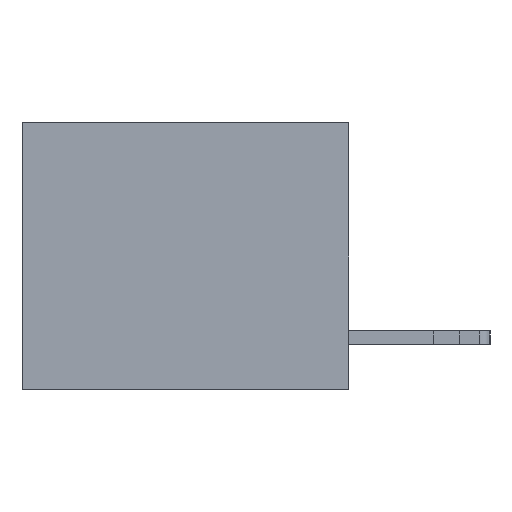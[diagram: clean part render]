
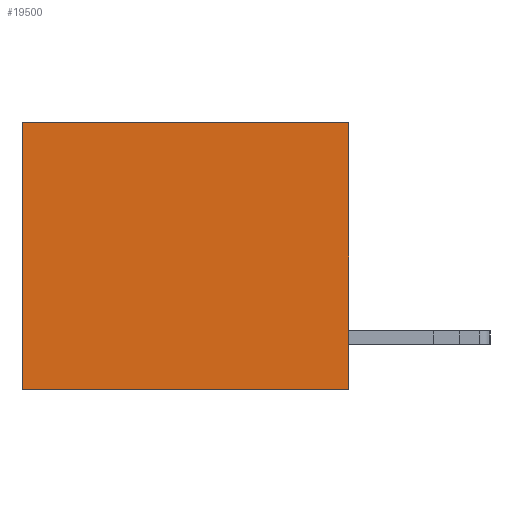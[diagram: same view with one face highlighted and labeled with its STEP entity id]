
A CAD part, left-side view. The second image highlights one B-rep face of the part: STEP entity #19500.
In plain terms, the highlighted planar face has unit normal (-1, 0, 0).
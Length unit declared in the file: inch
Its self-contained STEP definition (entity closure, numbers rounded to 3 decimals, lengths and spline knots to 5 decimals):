
#378 = DIRECTION ( 'NONE',  ( 0., 1., 0. ) ) ;
#2826 = DIRECTION ( 'NONE',  ( 1., 0., 0. ) ) ;
#3001 = CARTESIAN_POINT ( 'NONE',  ( 0.3165, 0.6, -0.49 ) ) ;
#3659 = VECTOR ( 'NONE', #4577, 39.37008 ) ;
#4577 = DIRECTION ( 'NONE',  ( 0., 0., -1. ) ) ;
#4807 = VECTOR ( 'NONE', #18859, 39.37008 ) ;
#5295 = CARTESIAN_POINT ( 'NONE',  ( 0.3165, 0.6, 0. ) ) ;
#5510 = CARTESIAN_POINT ( 'NONE',  ( 0.3165, 0., -0.49 ) ) ;
#6610 = LINE ( 'NONE', #30519, #25116 ) ;
#6663 = AXIS2_PLACEMENT_3D ( 'NONE', #5510, #2826, #17188 ) ;
#9792 = VERTEX_POINT ( 'NONE', #13735 ) ;
#12163 = LINE ( 'NONE', #23193, #4807 ) ;
#12301 = EDGE_CURVE ( 'NONE', #9792, #26466, #13832, .T. ) ;
#12869 = LINE ( 'NONE', #22359, #3659 ) ;
#13042 = ORIENTED_EDGE ( 'NONE', *, *, #18091, .T. ) ;
#13735 = CARTESIAN_POINT ( 'NONE',  ( 0.3165, 0., -0.49 ) ) ;
#13832 = LINE ( 'NONE', #24160, #20146 ) ;
#14188 = CARTESIAN_POINT ( 'NONE',  ( 0.3165, 0., 0. ) ) ;
#14693 = PLANE ( 'NONE',  #6663 ) ;
#14941 = VERTEX_POINT ( 'NONE', #14188 ) ;
#16459 = DIRECTION ( 'NONE',  ( 0., 0., -1. ) ) ;
#17188 = DIRECTION ( 'NONE',  ( 0., 0., -1. ) ) ;
#18091 = EDGE_CURVE ( 'NONE', #29698, #26466, #12869, .T. ) ;
#18859 = DIRECTION ( 'NONE',  ( 0., 1., 0. ) ) ;
#19500 = ADVANCED_FACE ( 'NONE', ( #27926 ), #14693, .F. ) ;
#19851 = EDGE_CURVE ( 'NONE', #14941, #29698, #12163, .T. ) ;
#19915 = EDGE_CURVE ( 'NONE', #14941, #9792, #6610, .T. ) ;
#20146 = VECTOR ( 'NONE', #378, 39.37008 ) ;
#22359 = CARTESIAN_POINT ( 'NONE',  ( 0.3165, 0.6, -0.49 ) ) ;
#23193 = CARTESIAN_POINT ( 'NONE',  ( 0.3165, 0., 0. ) ) ;
#24160 = CARTESIAN_POINT ( 'NONE',  ( 0.3165, 0., -0.49 ) ) ;
#25032 = ORIENTED_EDGE ( 'NONE', *, *, #19851, .T. ) ;
#25116 = VECTOR ( 'NONE', #16459, 39.37008 ) ;
#26466 = VERTEX_POINT ( 'NONE', #3001 ) ;
#27791 = EDGE_LOOP ( 'NONE', ( #13042, #28615, #29397, #25032 ) ) ;
#27926 = FACE_OUTER_BOUND ( 'NONE', #27791, .T. ) ;
#28615 = ORIENTED_EDGE ( 'NONE', *, *, #12301, .F. ) ;
#29397 = ORIENTED_EDGE ( 'NONE', *, *, #19915, .F. ) ;
#29698 = VERTEX_POINT ( 'NONE', #5295 ) ;
#30519 = CARTESIAN_POINT ( 'NONE',  ( 0.3165, 0., -0.49 ) ) ;
